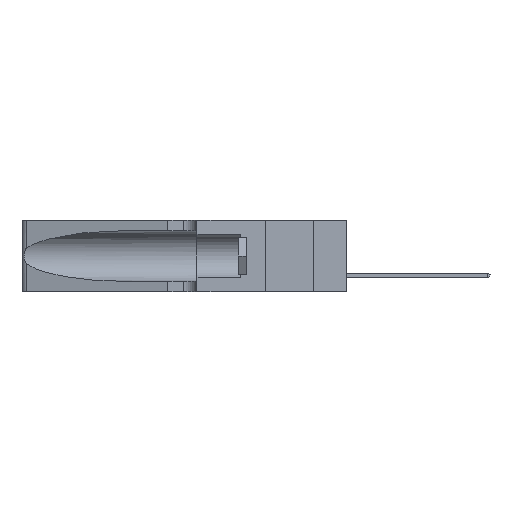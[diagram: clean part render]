
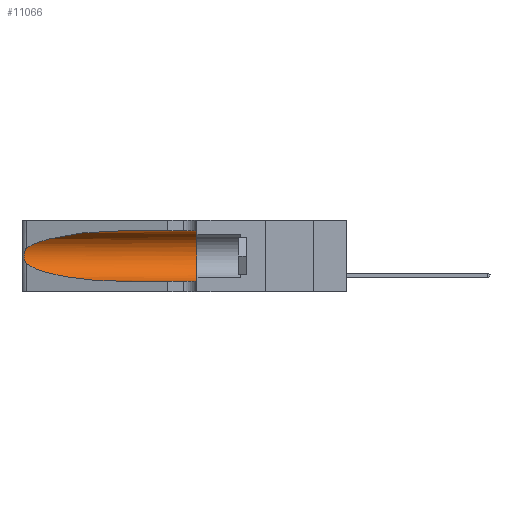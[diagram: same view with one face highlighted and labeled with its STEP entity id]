
A CAD part, left-side view. The second image highlights one B-rep face of the part: STEP entity #11066.
In plain terms, the highlighted cylindrical face has radius 3.308 mm (diameter 6.617 mm), a partial arc.
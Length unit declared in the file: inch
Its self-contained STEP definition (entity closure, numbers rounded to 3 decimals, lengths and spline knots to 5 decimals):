
#118 = CARTESIAN_POINT ( 'NONE',  ( 0.25639, 1.23184, 0.21858 ) ) ;
#432 = CARTESIAN_POINT ( 'NONE',  ( 0.1305, 0.35, 0.185 ) ) ;
#738 = AXIS2_PLACEMENT_3D ( 'NONE', #432, #2569, #7419 ) ;
#1419 = CARTESIAN_POINT ( 'NONE',  ( 0.1305, 0.72297, 0.31525 ) ) ;
#1435 = CARTESIAN_POINT ( 'NONE',  ( 0.1305, 0.35, 0.05475 ) ) ;
#2080 = CARTESIAN_POINT ( 'NONE',  ( 0.18966, 0.96281, 0.05475 ) ) ;
#2085 = CARTESIAN_POINT ( 'NONE',  ( 0.1305, 1.61858, 0.05475 ) ) ;
#2189 = FACE_OUTER_BOUND ( 'NONE', #26350, .T. ) ;
#2559 = CARTESIAN_POINT ( 'NONE',  ( 0.26017, 1.23833, 0.17102 ) ) ;
#2569 = DIRECTION ( 'NONE',  ( 0., 1., 0. ) ) ;
#2660 = CARTESIAN_POINT ( 'NONE',  ( 0.25789, 1.23486, 0.15765 ) ) ;
#2956 = CARTESIAN_POINT ( 'NONE',  ( 0.25487, 1.22718, 0.14631 ) ) ;
#4238 = EDGE_CURVE ( 'NONE', #19852, #7121, #27312, .T. ) ;
#4722 = DIRECTION ( 'NONE',  ( 0., -1., 0. ) ) ;
#4974 = CARTESIAN_POINT ( 'NONE',  ( 0.25639, 1.23186, 0.15144 ) ) ;
#5987 = CARTESIAN_POINT ( 'NONE',  ( 0.1305, 0.72297, 0.31525 ) ) ;
#6530 = LINE ( 'NONE', #21869, #16725 ) ;
#6908 = VECTOR ( 'NONE', #4722, 39.37008 ) ;
#7121 = VERTEX_POINT ( 'NONE', #1435 ) ;
#7214 = CARTESIAN_POINT ( 'NONE',  ( 0.25487, 1.22718, 0.22369 ) ) ;
#7316 = CARTESIAN_POINT ( 'NONE',  ( 0.26075, 1.23896, 0.19203 ) ) ;
#7419 = DIRECTION ( 'NONE',  ( 0., 0., 1. ) ) ;
#7519 = CARTESIAN_POINT ( 'NONE',  ( 0.25555, 1.22994, 0.2215 ) ) ;
#7678 = ORIENTED_EDGE ( 'NONE', *, *, #12030, .T. ) ;
#9035 = EDGE_CURVE ( 'NONE', #9108, #26952, #23431, .T. ) ;
#9108 = VERTEX_POINT ( 'NONE', #16398 ) ;
#9700 = CARTESIAN_POINT ( 'NONE',  ( 0.1305, 1.61858, 0.185 ) ) ;
#11020 = EDGE_CURVE ( 'NONE', #26952, #7121, #14605, .T. ) ;
#11066 = ADVANCED_FACE ( 'NONE', ( #2189 ), #23929, .F. ) ;
#11829 = CARTESIAN_POINT ( 'NONE',  ( 0.25787, 1.23484, 0.2124 ) ) ;
#12030 = EDGE_CURVE ( 'NONE', #27180, #24214, #13674, .T. ) ;
#12031 = ORIENTED_EDGE ( 'NONE', *, *, #9035, .T. ) ;
#13591 = EDGE_CURVE ( 'NONE', #24214, #9108, #27481, .T. ) ;
#13674 =( BOUNDED_CURVE ( )  B_SPLINE_CURVE ( 3, ( #1419, #17661, #17472, #22201 ),
 .UNSPECIFIED., .F., .T. ) 
 B_SPLINE_CURVE_WITH_KNOTS ( ( 4, 4 ),
 ( 1.5708, 2.84003 ),
 .UNSPECIFIED. ) 
 CURVE ( )  GEOMETRIC_REPRESENTATION_ITEM ( )  RATIONAL_B_SPLINE_CURVE ( ( 1., 0.87, 0.87, 1. ) ) 
 REPRESENTATION_ITEM ( '' )  );
#14194 = CARTESIAN_POINT ( 'NONE',  ( 0.26018, 1.23835, 0.19895 ) ) ;
#14605 = LINE ( 'NONE', #2085, #6908 ) ;
#16398 = CARTESIAN_POINT ( 'NONE',  ( 0.25487, 1.22718, 0.14631 ) ) ;
#16473 = CARTESIAN_POINT ( 'NONE',  ( 0.26075, 1.23896, 0.178 ) ) ;
#16725 = VECTOR ( 'NONE', #17430, 39.37008 ) ;
#17430 = DIRECTION ( 'NONE',  ( 0., -1., 0. ) ) ;
#17472 = CARTESIAN_POINT ( 'NONE',  ( 0.2373, 1.15595, 0.28018 ) ) ;
#17661 = CARTESIAN_POINT ( 'NONE',  ( 0.18966, 0.96281, 0.31525 ) ) ;
#18436 = AXIS2_PLACEMENT_3D ( 'NONE', #9700, #21343, #21149 ) ;
#18785 = CARTESIAN_POINT ( 'NONE',  ( 0.25856, 1.23593, 0.16098 ) ) ;
#19852 = VERTEX_POINT ( 'NONE', #20970 ) ;
#20486 = EDGE_CURVE ( 'NONE', #27180, #19852, #6530, .T. ) ;
#20970 = CARTESIAN_POINT ( 'NONE',  ( 0.1305, 0.35, 0.31525 ) ) ;
#21149 = DIRECTION ( 'NONE',  ( 0., 0., -1. ) ) ;
#21343 = DIRECTION ( 'NONE',  ( 0., -1., 0. ) ) ;
#21530 = CARTESIAN_POINT ( 'NONE',  ( 0.25487, 1.22718, 0.22369 ) ) ;
#21869 = CARTESIAN_POINT ( 'NONE',  ( 0.1305, 1.61858, 0.31525 ) ) ;
#22201 = CARTESIAN_POINT ( 'NONE',  ( 0.25487, 1.22718, 0.22369 ) ) ;
#22565 = ORIENTED_EDGE ( 'NONE', *, *, #13591, .T. ) ;
#23130 = ORIENTED_EDGE ( 'NONE', *, *, #11020, .T. ) ;
#23431 =( BOUNDED_CURVE ( )  B_SPLINE_CURVE ( 3, ( #25023, #29702, #2080, #27355 ),
 .UNSPECIFIED., .F., .F. ) 
 B_SPLINE_CURVE_WITH_KNOTS ( ( 4, 4 ),
 ( 3.44316, 4.71239 ),
 .UNSPECIFIED. ) 
 CURVE ( )  GEOMETRIC_REPRESENTATION_ITEM ( )  RATIONAL_B_SPLINE_CURVE ( ( 1., 0.87, 0.87, 1. ) ) 
 REPRESENTATION_ITEM ( '' )  );
#23508 = CARTESIAN_POINT ( 'NONE',  ( 0.25555, 1.22993, 0.14849 ) ) ;
#23929 = CYLINDRICAL_SURFACE ( 'NONE', #18436, 0.13025 ) ;
#24214 = VERTEX_POINT ( 'NONE', #21530 ) ;
#25023 = CARTESIAN_POINT ( 'NONE',  ( 0.25487, 1.22718, 0.14631 ) ) ;
#26350 = EDGE_LOOP ( 'NONE', ( #7678, #22565, #12031, #23130, #29588, #28811 ) ) ;
#26952 = VERTEX_POINT ( 'NONE', #28456 ) ;
#27180 = VERTEX_POINT ( 'NONE', #5987 ) ;
#27312 = CIRCLE ( 'NONE', #738, 0.13025 ) ;
#27355 = CARTESIAN_POINT ( 'NONE',  ( 0.1305, 0.72297, 0.05475 ) ) ;
#27481 = B_SPLINE_CURVE_WITH_KNOTS ( 'NONE', 3,
 ( #7214, #7519, #118, #11829, #27954, #14194, #7316, #16473, #2559, #18785, #2660, #4974, #23508, #2956 ),
 .UNSPECIFIED., .F., .F.,
 ( 4, 2, 2, 2, 2, 2, 4 ),
 ( 0., 0.00027, 0.00053, 0.00107, 0.0016, 0.00187, 0.00214 ),
 .UNSPECIFIED. ) ;
#27954 = CARTESIAN_POINT ( 'NONE',  ( 0.25854, 1.2359, 0.20912 ) ) ;
#28456 = CARTESIAN_POINT ( 'NONE',  ( 0.1305, 0.72297, 0.05475 ) ) ;
#28811 = ORIENTED_EDGE ( 'NONE', *, *, #20486, .F. ) ;
#29588 = ORIENTED_EDGE ( 'NONE', *, *, #4238, .F. ) ;
#29702 = CARTESIAN_POINT ( 'NONE',  ( 0.2373, 1.15595, 0.08982 ) ) ;
